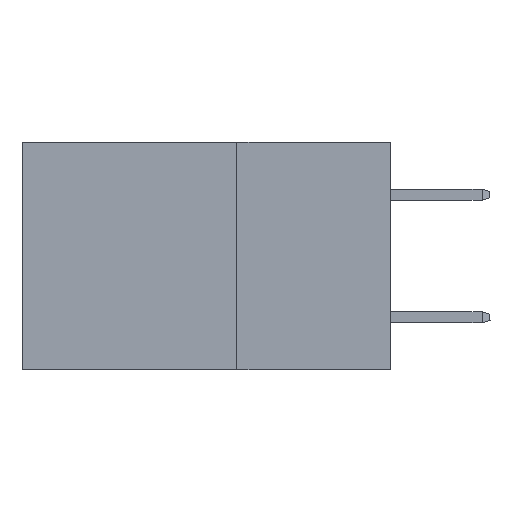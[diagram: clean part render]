
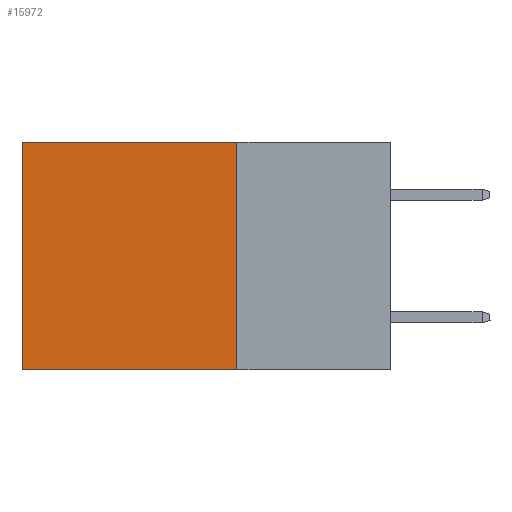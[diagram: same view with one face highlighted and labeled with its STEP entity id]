
A CAD part, left-side view. The second image highlights one B-rep face of the part: STEP entity #15972.
In plain terms, the highlighted planar face has unit normal (-1, 0, 0).
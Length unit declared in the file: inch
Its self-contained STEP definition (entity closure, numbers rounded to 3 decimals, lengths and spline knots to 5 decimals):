
#47 = ORIENTED_EDGE ( 'NONE', *, *, #20776, .F. ) ;
#946 = LINE ( 'NONE', #5176, #15075 ) ;
#1548 = EDGE_LOOP ( 'NONE', ( #3900, #47, #20748, #6113 ) ) ;
#1558 = DIRECTION ( 'NONE',  ( 0., 0., -1. ) ) ;
#2099 = LINE ( 'NONE', #19183, #5819 ) ;
#3182 = VERTEX_POINT ( 'NONE', #12533 ) ;
#3900 = ORIENTED_EDGE ( 'NONE', *, *, #19381, .T. ) ;
#4938 = CARTESIAN_POINT ( 'NONE',  ( 0.2875, 0.25, 0. ) ) ;
#5176 = CARTESIAN_POINT ( 'NONE',  ( 0.2875, 0.25, 0. ) ) ;
#5819 = VECTOR ( 'NONE', #6953, 39.37008 ) ;
#6113 = ORIENTED_EDGE ( 'NONE', *, *, #6466, .T. ) ;
#6466 = EDGE_CURVE ( 'NONE', #22461, #3182, #2099, .T. ) ;
#6472 = EDGE_CURVE ( 'NONE', #22461, #6663, #946, .T. ) ;
#6663 = VERTEX_POINT ( 'NONE', #21373 ) ;
#6953 = DIRECTION ( 'NONE',  ( 0., 1., 0. ) ) ;
#6955 = CARTESIAN_POINT ( 'NONE',  ( 0.2875, 0.6, 0. ) ) ;
#8501 = DIRECTION ( 'NONE',  ( 0., 1., 0. ) ) ;
#9846 = CARTESIAN_POINT ( 'NONE',  ( 0.2875, 0.6, -0.37 ) ) ;
#10005 = LINE ( 'NONE', #22567, #14073 ) ;
#10497 = PLANE ( 'NONE',  #19464 ) ;
#12230 = DIRECTION ( 'NONE',  ( 0., 0., -1. ) ) ;
#12241 = DIRECTION ( 'NONE',  ( 1., 0., 0. ) ) ;
#12423 = FACE_OUTER_BOUND ( 'NONE', #1548, .T. ) ;
#12533 = CARTESIAN_POINT ( 'NONE',  ( 0.2875, 0.6, 0. ) ) ;
#12557 = VECTOR ( 'NONE', #12230, 39.37008 ) ;
#13088 = LINE ( 'NONE', #6955, #12557 ) ;
#14073 = VECTOR ( 'NONE', #8501, 39.37008 ) ;
#15075 = VECTOR ( 'NONE', #15612, 39.37008 ) ;
#15612 = DIRECTION ( 'NONE',  ( 0., 0., -1. ) ) ;
#15626 = CARTESIAN_POINT ( 'NONE',  ( 0.2875, 0.25, 0. ) ) ;
#15972 = ADVANCED_FACE ( 'NONE', ( #12423 ), #10497, .F. ) ;
#17864 = VERTEX_POINT ( 'NONE', #9846 ) ;
#19183 = CARTESIAN_POINT ( 'NONE',  ( 0.2875, 0.25, 0. ) ) ;
#19381 = EDGE_CURVE ( 'NONE', #3182, #17864, #13088, .T. ) ;
#19464 = AXIS2_PLACEMENT_3D ( 'NONE', #15626, #12241, #1558 ) ;
#20748 = ORIENTED_EDGE ( 'NONE', *, *, #6472, .F. ) ;
#20776 = EDGE_CURVE ( 'NONE', #6663, #17864, #10005, .T. ) ;
#21373 = CARTESIAN_POINT ( 'NONE',  ( 0.2875, 0.25, -0.37 ) ) ;
#22461 = VERTEX_POINT ( 'NONE', #4938 ) ;
#22567 = CARTESIAN_POINT ( 'NONE',  ( 0.2875, 0.25, -0.37 ) ) ;
